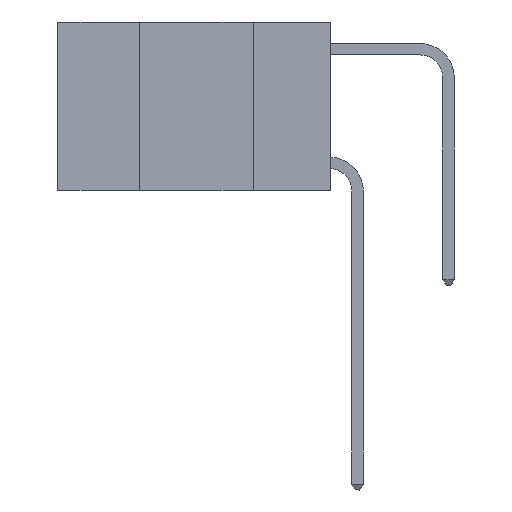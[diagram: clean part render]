
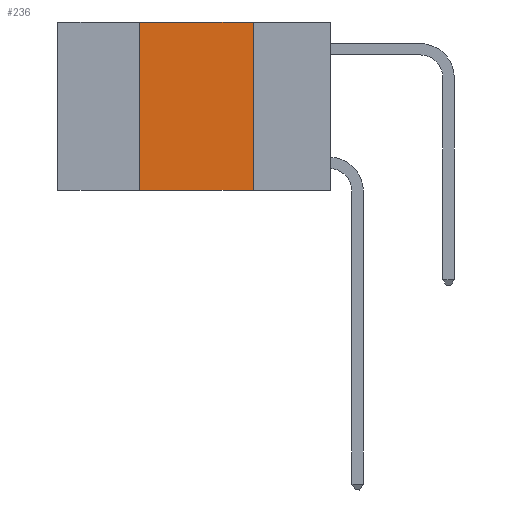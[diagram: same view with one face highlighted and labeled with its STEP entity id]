
A CAD part, left-side view. The second image highlights one B-rep face of the part: STEP entity #236.
In plain terms, the highlighted planar face has unit normal (-1, 0, 0).
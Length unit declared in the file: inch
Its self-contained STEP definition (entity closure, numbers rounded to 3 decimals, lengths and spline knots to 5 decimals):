
#236 = ADVANCED_FACE ( 'NONE', ( #1430 ), #10068, .F. ) ;
#449 = CARTESIAN_POINT ( 'NONE',  ( 0., 0.17, -0.37 ) ) ;
#682 = EDGE_CURVE ( 'NONE', #7703, #6902, #8558, .T. ) ;
#1429 = LINE ( 'NONE', #8888, #6576 ) ;
#1430 = FACE_OUTER_BOUND ( 'NONE', #6127, .T. ) ;
#1973 = VECTOR ( 'NONE', #3689, 39.37008 ) ;
#2042 = EDGE_CURVE ( 'NONE', #10531, #2646, #1429, .T. ) ;
#2057 = EDGE_CURVE ( 'NONE', #7703, #10531, #7527, .T. ) ;
#2295 = CARTESIAN_POINT ( 'NONE',  ( 0., 0.42, 0. ) ) ;
#2646 = VERTEX_POINT ( 'NONE', #5652 ) ;
#2964 = ORIENTED_EDGE ( 'NONE', *, *, #2042, .F. ) ;
#3364 = CARTESIAN_POINT ( 'NONE',  ( 0., 0.6, -0.37 ) ) ;
#3521 = ORIENTED_EDGE ( 'NONE', *, *, #9629, .F. ) ;
#3689 = DIRECTION ( 'NONE',  ( 0., 0., -1. ) ) ;
#3764 = DIRECTION ( 'NONE',  ( 0., -1., 0. ) ) ;
#5082 = AXIS2_PLACEMENT_3D ( 'NONE', #10934, #7330, #10968 ) ;
#5294 = VECTOR ( 'NONE', #6835, 39.37008 ) ;
#5605 = DIRECTION ( 'NONE',  ( 0., 0., 1. ) ) ;
#5652 = CARTESIAN_POINT ( 'NONE',  ( 0., 0.17, 0. ) ) ;
#6127 = EDGE_LOOP ( 'NONE', ( #3521, #2964, #9644, #9714 ) ) ;
#6384 = LINE ( 'NONE', #7011, #1973 ) ;
#6576 = VECTOR ( 'NONE', #3764, 39.37008 ) ;
#6835 = DIRECTION ( 'NONE',  ( 0., -1., 0. ) ) ;
#6902 = VERTEX_POINT ( 'NONE', #449 ) ;
#7011 = CARTESIAN_POINT ( 'NONE',  ( 0., 0.17, 0. ) ) ;
#7129 = VECTOR ( 'NONE', #5605, 39.37008 ) ;
#7330 = DIRECTION ( 'NONE',  ( 1., 0., 0. ) ) ;
#7527 = LINE ( 'NONE', #2295, #7129 ) ;
#7703 = VERTEX_POINT ( 'NONE', #10381 ) ;
#7971 = CARTESIAN_POINT ( 'NONE',  ( 0., 0.42, 0. ) ) ;
#8558 = LINE ( 'NONE', #3364, #5294 ) ;
#8888 = CARTESIAN_POINT ( 'NONE',  ( 0., 0.6, 0. ) ) ;
#9629 = EDGE_CURVE ( 'NONE', #2646, #6902, #6384, .T. ) ;
#9644 = ORIENTED_EDGE ( 'NONE', *, *, #2057, .F. ) ;
#9714 = ORIENTED_EDGE ( 'NONE', *, *, #682, .T. ) ;
#10068 = PLANE ( 'NONE',  #5082 ) ;
#10381 = CARTESIAN_POINT ( 'NONE',  ( 0., 0.42, -0.37 ) ) ;
#10531 = VERTEX_POINT ( 'NONE', #7971 ) ;
#10934 = CARTESIAN_POINT ( 'NONE',  ( 0., 0.6, 0. ) ) ;
#10968 = DIRECTION ( 'NONE',  ( 0., 0., -1. ) ) ;
